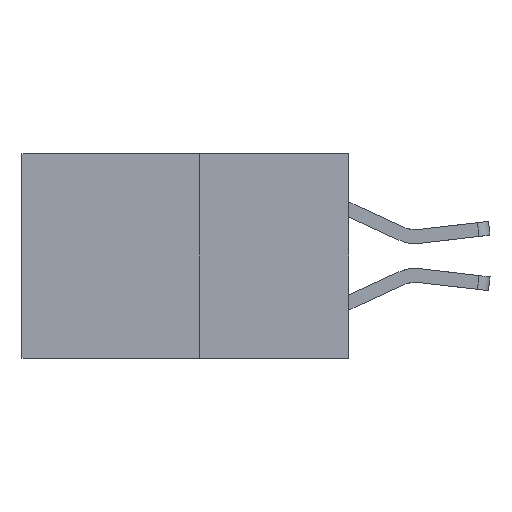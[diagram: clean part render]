
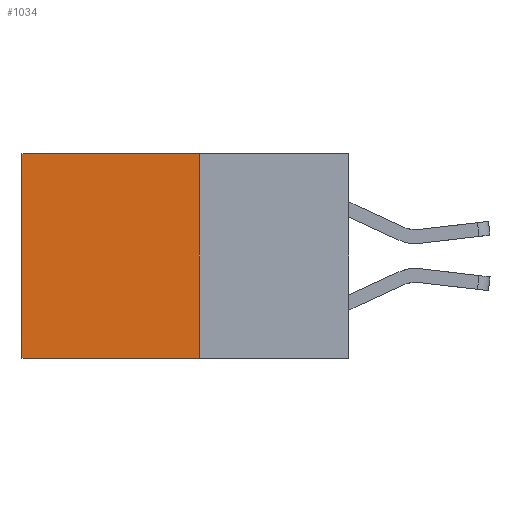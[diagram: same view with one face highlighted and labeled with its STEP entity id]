
A CAD part, left-side view. The second image highlights one B-rep face of the part: STEP entity #1034.
In plain terms, the highlighted planar face has unit normal (-1, 0, 0).
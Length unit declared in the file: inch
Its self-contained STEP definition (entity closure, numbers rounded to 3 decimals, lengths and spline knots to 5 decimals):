
#52 = CARTESIAN_POINT ( 'NONE',  ( 0.277, 0.59, -0.37 ) ) ;
#188 = VECTOR ( 'NONE', #996, 39.37008 ) ;
#375 = EDGE_CURVE ( 'NONE', #2432, #2700, #6474, .T. ) ;
#996 = DIRECTION ( 'NONE',  ( 0., 0., -1. ) ) ;
#1034 = ADVANCED_FACE ( 'NONE', ( #5839 ), #6040, .F. ) ;
#1046 = ORIENTED_EDGE ( 'NONE', *, *, #2021, .F. ) ;
#1060 = CARTESIAN_POINT ( 'NONE',  ( 0.277, 0.59, 0. ) ) ;
#1464 = VECTOR ( 'NONE', #5787, 39.37008 ) ;
#1932 = CARTESIAN_POINT ( 'NONE',  ( 0.277, 0.59, -0.37 ) ) ;
#2021 = EDGE_CURVE ( 'NONE', #4465, #2700, #5323, .T. ) ;
#2432 = VERTEX_POINT ( 'NONE', #1060 ) ;
#2626 = VECTOR ( 'NONE', #6267, 39.37008 ) ;
#2700 = VERTEX_POINT ( 'NONE', #52 ) ;
#3225 = CARTESIAN_POINT ( 'NONE',  ( 0.277, 0.27, -0.37 ) ) ;
#4110 = CARTESIAN_POINT ( 'NONE',  ( 0.277, 0.27, -0.37 ) ) ;
#4410 = EDGE_CURVE ( 'NONE', #8989, #4465, #8550, .T. ) ;
#4449 = DIRECTION ( 'NONE',  ( 1., 0., 0. ) ) ;
#4465 = VERTEX_POINT ( 'NONE', #4110 ) ;
#4659 = LINE ( 'NONE', #5483, #2626 ) ;
#5025 = CARTESIAN_POINT ( 'NONE',  ( 0.277, 0.27, 0. ) ) ;
#5280 = DIRECTION ( 'NONE',  ( 0., 0., -1. ) ) ;
#5323 = LINE ( 'NONE', #5796, #1464 ) ;
#5483 = CARTESIAN_POINT ( 'NONE',  ( 0.277, 0.27, 0. ) ) ;
#5607 = CARTESIAN_POINT ( 'NONE',  ( 0.277, 0.27, -0.37 ) ) ;
#5787 = DIRECTION ( 'NONE',  ( 0., 1., 0. ) ) ;
#5796 = CARTESIAN_POINT ( 'NONE',  ( 0.277, 0.27, -0.37 ) ) ;
#5839 = FACE_OUTER_BOUND ( 'NONE', #6611, .T. ) ;
#5918 = ORIENTED_EDGE ( 'NONE', *, *, #375, .T. ) ;
#6040 = PLANE ( 'NONE',  #8553 ) ;
#6227 = VECTOR ( 'NONE', #5280, 39.37008 ) ;
#6267 = DIRECTION ( 'NONE',  ( 0., 1., 0. ) ) ;
#6361 = EDGE_CURVE ( 'NONE', #8989, #2432, #4659, .T. ) ;
#6474 = LINE ( 'NONE', #1932, #6227 ) ;
#6611 = EDGE_LOOP ( 'NONE', ( #5918, #1046, #9573, #7473 ) ) ;
#7473 = ORIENTED_EDGE ( 'NONE', *, *, #6361, .T. ) ;
#8550 = LINE ( 'NONE', #5607, #188 ) ;
#8553 = AXIS2_PLACEMENT_3D ( 'NONE', #3225, #4449, #9607 ) ;
#8989 = VERTEX_POINT ( 'NONE', #5025 ) ;
#9573 = ORIENTED_EDGE ( 'NONE', *, *, #4410, .F. ) ;
#9607 = DIRECTION ( 'NONE',  ( 0., 0., -1. ) ) ;
